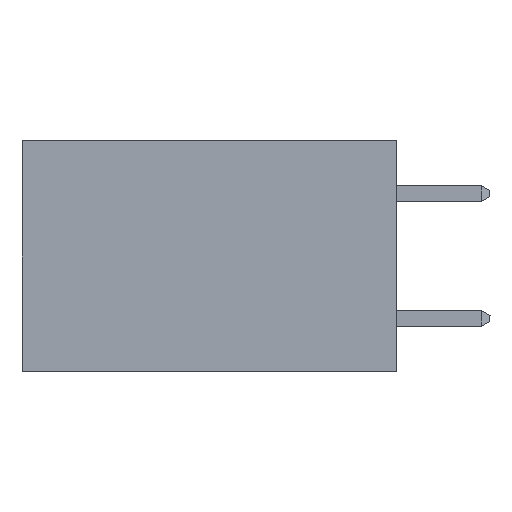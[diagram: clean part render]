
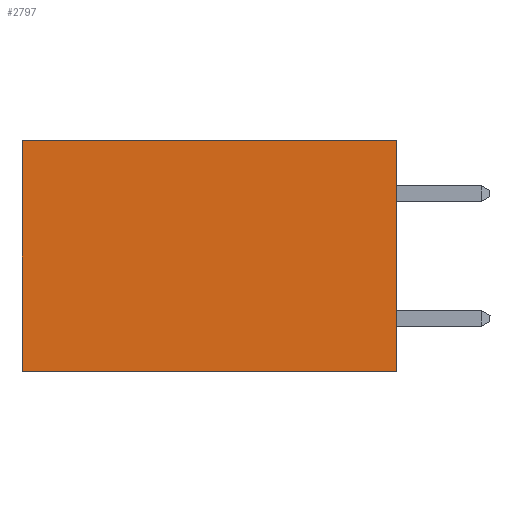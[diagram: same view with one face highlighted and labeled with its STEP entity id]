
A CAD part, left-side view. The second image highlights one B-rep face of the part: STEP entity #2797.
In plain terms, the highlighted planar face has unit normal (-1, 0, 0).
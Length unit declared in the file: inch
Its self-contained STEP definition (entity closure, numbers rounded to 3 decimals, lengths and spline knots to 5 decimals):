
#26 = LINE ( 'NONE', #4551, #12166 ) ;
#572 = VERTEX_POINT ( 'NONE', #8896 ) ;
#1225 = DIRECTION ( 'NONE',  ( 1., 0., 0. ) ) ;
#1247 = DIRECTION ( 'NONE',  ( 0., 0., -1. ) ) ;
#1722 = EDGE_LOOP ( 'NONE', ( #2515, #2863, #4501, #8260 ) ) ;
#1751 = FACE_OUTER_BOUND ( 'NONE', #1722, .T. ) ;
#1978 = CARTESIAN_POINT ( 'NONE',  ( 0.2615, 0., 0. ) ) ;
#2219 = EDGE_CURVE ( 'NONE', #10032, #572, #8933, .T. ) ;
#2515 = ORIENTED_EDGE ( 'NONE', *, *, #3621, .T. ) ;
#2797 = ADVANCED_FACE ( 'NONE', ( #1751 ), #10076, .F. ) ;
#2863 = ORIENTED_EDGE ( 'NONE', *, *, #5348, .F. ) ;
#3127 = EDGE_CURVE ( 'NONE', #10032, #3192, #6117, .T. ) ;
#3192 = VERTEX_POINT ( 'NONE', #12388 ) ;
#3544 = VERTEX_POINT ( 'NONE', #12020 ) ;
#3621 = EDGE_CURVE ( 'NONE', #3192, #3544, #11118, .T. ) ;
#3963 = DIRECTION ( 'NONE',  ( 0., 1., 0. ) ) ;
#4501 = ORIENTED_EDGE ( 'NONE', *, *, #2219, .F. ) ;
#4551 = CARTESIAN_POINT ( 'NONE',  ( 0.2615, 0., -0.37 ) ) ;
#4888 = DIRECTION ( 'NONE',  ( 0., 1., 0. ) ) ;
#5023 = DIRECTION ( 'NONE',  ( 0., 0., -1. ) ) ;
#5149 = CARTESIAN_POINT ( 'NONE',  ( 0.2615, 0., -0.37 ) ) ;
#5348 = EDGE_CURVE ( 'NONE', #572, #3544, #26, .T. ) ;
#6117 = LINE ( 'NONE', #1978, #11173 ) ;
#7014 = CARTESIAN_POINT ( 'NONE',  ( 0.2615, 0., 0. ) ) ;
#8260 = ORIENTED_EDGE ( 'NONE', *, *, #3127, .T. ) ;
#8627 = VECTOR ( 'NONE', #5023, 39.37008 ) ;
#8896 = CARTESIAN_POINT ( 'NONE',  ( 0.2615, 0., -0.37 ) ) ;
#8933 = LINE ( 'NONE', #5149, #8627 ) ;
#10032 = VERTEX_POINT ( 'NONE', #7014 ) ;
#10076 = PLANE ( 'NONE',  #11789 ) ;
#10333 = CARTESIAN_POINT ( 'NONE',  ( 0.2615, 0., -0.37 ) ) ;
#10594 = DIRECTION ( 'NONE',  ( 0., 0., -1. ) ) ;
#10603 = CARTESIAN_POINT ( 'NONE',  ( 0.2615, 0.6, -0.37 ) ) ;
#11118 = LINE ( 'NONE', #10603, #11378 ) ;
#11173 = VECTOR ( 'NONE', #3963, 39.37008 ) ;
#11378 = VECTOR ( 'NONE', #10594, 39.37008 ) ;
#11789 = AXIS2_PLACEMENT_3D ( 'NONE', #10333, #1225, #1247 ) ;
#12020 = CARTESIAN_POINT ( 'NONE',  ( 0.2615, 0.6, -0.37 ) ) ;
#12166 = VECTOR ( 'NONE', #4888, 39.37008 ) ;
#12388 = CARTESIAN_POINT ( 'NONE',  ( 0.2615, 0.6, 0. ) ) ;
